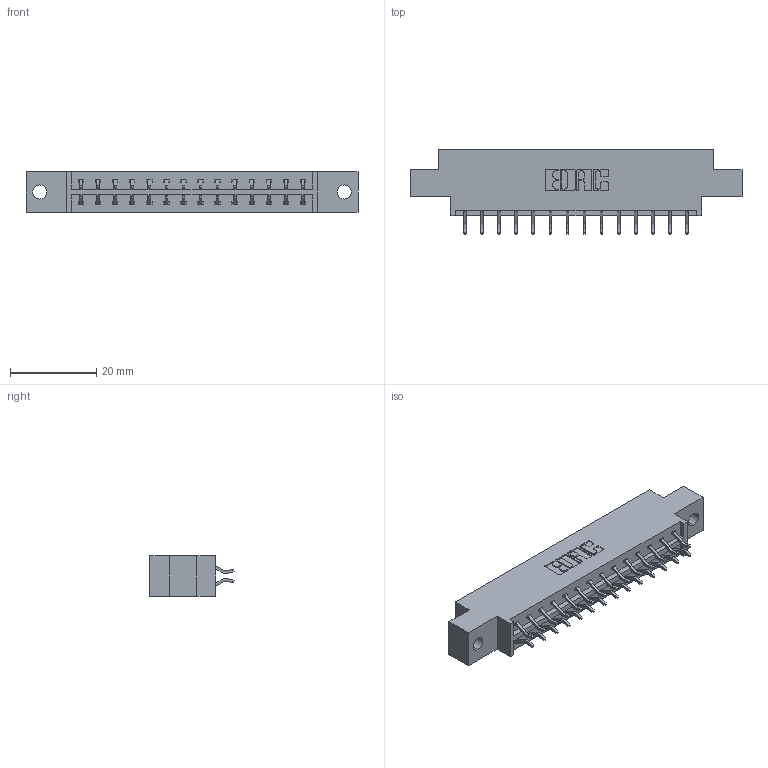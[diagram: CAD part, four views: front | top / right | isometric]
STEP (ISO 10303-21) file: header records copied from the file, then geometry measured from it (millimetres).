
FILE_DESCRIPTION (( 'STEP AP203' ), '1' );
FILE_NAME ('333-028-556-802.STEP', '2018-08-02T15:41:59', ( '' ), ( '' ), 'SwSTEP 2.0', 'SolidWorks 2016', '' );
FILE_SCHEMA (( 'CONFIG_CONTROL_DESIGN' ));
Length unit declared in the file: inch
Products named in the file (3): 333-028-556-802; 333 Part_Offset - .128 Dia; 345-292-001_556 Tail
Assembly tree (29 placements, depth 2):
  333-028-556-802
    333 Part_Offset - .128 Dia
    345-292-001_556 Tail  x28
Bounding box: 77.01 x 19.57 x 9.4 mm (x, y, z)
Volume: 7335.1 mm3; surface area: 8291 mm2
Topology: 29 solids, 29 shells, 1742 faces, 5167 edges, 3406 vertices
Faces by surface type: plane 1194, cylinder 548
Entity records: 12983 total; most frequent: CARTESIAN_POINT 2202, ORIENTED_EDGE 2126, DIRECTION 1919, EDGE_CURVE 1063, LINE 927, VECTOR 927, VERTEX_POINT 706, AXIS2_PLACEMENT_3D 496
